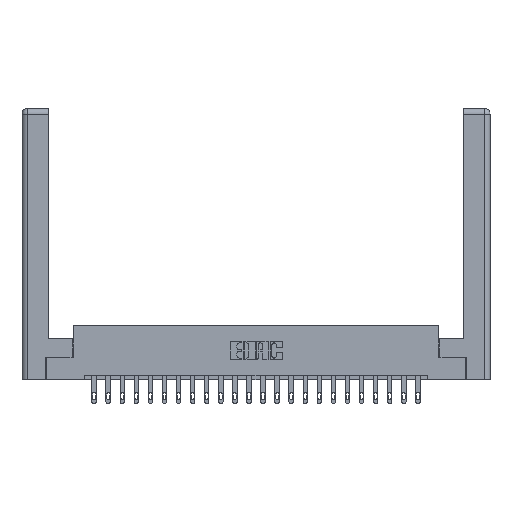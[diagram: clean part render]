
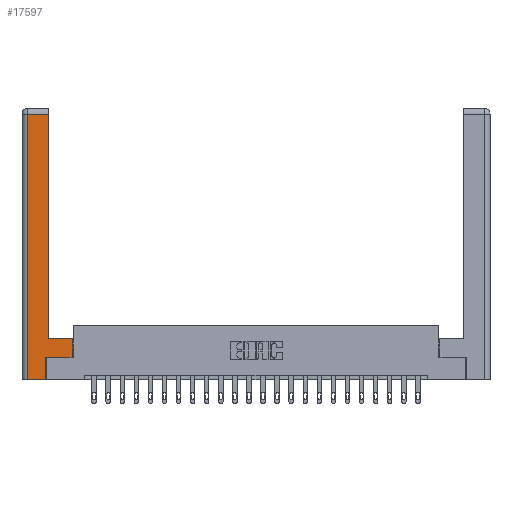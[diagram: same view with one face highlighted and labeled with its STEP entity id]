
A CAD part, top view. The second image highlights one B-rep face of the part: STEP entity #17597.
In plain terms, the highlighted planar face has unit normal (0, 0, 1).
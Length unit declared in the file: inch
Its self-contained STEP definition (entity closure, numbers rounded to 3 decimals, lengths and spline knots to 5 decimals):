
#208 = VECTOR ( 'NONE', #2813, 39.37008 ) ;
#710 = CARTESIAN_POINT ( 'NONE',  ( 0.565, 0.45, 0. ) ) ;
#1261 = VECTOR ( 'NONE', #11928, 39.37008 ) ;
#1658 = VERTEX_POINT ( 'NONE', #710 ) ;
#2043 = LINE ( 'NONE', #23170, #2915 ) ;
#2446 = DIRECTION ( 'NONE',  ( 0., 1., 0. ) ) ;
#2464 = VERTEX_POINT ( 'NONE', #9909 ) ;
#2813 = DIRECTION ( 'NONE',  ( 0., 1., 0. ) ) ;
#2915 = VECTOR ( 'NONE', #17894, 39.37008 ) ;
#3026 = EDGE_LOOP ( 'NONE', ( #8610, #19507, #13504, #21612, #8413, #15944, #18445, #5340 ) ) ;
#3492 = LINE ( 'NONE', #3715, #17320 ) ;
#3670 = VERTEX_POINT ( 'NONE', #4902 ) ;
#3715 = CARTESIAN_POINT ( 'NONE',  ( 0.265, 0., 0. ) ) ;
#3839 = EDGE_CURVE ( 'NONE', #1658, #21375, #17519, .T. ) ;
#3947 = CARTESIAN_POINT ( 'NONE',  ( 0.565, 0.45, 0. ) ) ;
#4124 = CARTESIAN_POINT ( 'NONE',  ( 0.295, 0.45, 0. ) ) ;
#4676 = LINE ( 'NONE', #12183, #22769 ) ;
#4801 = DIRECTION ( 'NONE',  ( -1., 0., 0. ) ) ;
#4902 = CARTESIAN_POINT ( 'NONE',  ( 0.295, 2.94, 0. ) ) ;
#5340 = ORIENTED_EDGE ( 'NONE', *, *, #3839, .T. ) ;
#5604 = CARTESIAN_POINT ( 'NONE',  ( 0.295, 0.45, 0. ) ) ;
#6064 = EDGE_CURVE ( 'NONE', #7318, #17657, #23118, .T. ) ;
#6409 = VERTEX_POINT ( 'NONE', #15928 ) ;
#6673 = DIRECTION ( 'NONE',  ( 1., 0., 0. ) ) ;
#6937 = VECTOR ( 'NONE', #2446, 39.37008 ) ;
#7318 = VERTEX_POINT ( 'NONE', #20897 ) ;
#7403 = FACE_OUTER_BOUND ( 'NONE', #3026, .T. ) ;
#8309 = CARTESIAN_POINT ( 'NONE',  ( 0.0615, 0., 0. ) ) ;
#8355 = EDGE_CURVE ( 'NONE', #2464, #1658, #20774, .T. ) ;
#8413 = ORIENTED_EDGE ( 'NONE', *, *, #6064, .T. ) ;
#8610 = ORIENTED_EDGE ( 'NONE', *, *, #10996, .T. ) ;
#9100 = EDGE_CURVE ( 'NONE', #6409, #7318, #3492, .T. ) ;
#9909 = CARTESIAN_POINT ( 'NONE',  ( 0.565, 0.245, 0. ) ) ;
#10368 = PLANE ( 'NONE',  #14100 ) ;
#10924 = LINE ( 'NONE', #8309, #1261 ) ;
#10996 = EDGE_CURVE ( 'NONE', #21375, #3670, #20335, .T. ) ;
#11390 = VECTOR ( 'NONE', #12776, 39.37008 ) ;
#11513 = CARTESIAN_POINT ( 'NONE',  ( 0., 0., 0. ) ) ;
#11928 = DIRECTION ( 'NONE',  ( 0., -1., 0. ) ) ;
#12183 = CARTESIAN_POINT ( 'NONE',  ( 0.0615, 2.94, 0. ) ) ;
#12776 = DIRECTION ( 'NONE',  ( 0., 1., 0. ) ) ;
#12834 = DIRECTION ( 'NONE',  ( 0., 0., -1. ) ) ;
#13333 = CARTESIAN_POINT ( 'NONE',  ( 0.295, 3., 0. ) ) ;
#13504 = ORIENTED_EDGE ( 'NONE', *, *, #20270, .T. ) ;
#13834 = CARTESIAN_POINT ( 'NONE',  ( 0.0615, 2.94, 0. ) ) ;
#14100 = AXIS2_PLACEMENT_3D ( 'NONE', #11513, #12834, #4801 ) ;
#15358 = CARTESIAN_POINT ( 'NONE',  ( 0.265, 0.245, 0. ) ) ;
#15503 = EDGE_CURVE ( 'NONE', #17657, #2464, #2043, .T. ) ;
#15928 = CARTESIAN_POINT ( 'NONE',  ( 0.0615, 0., 0. ) ) ;
#15944 = ORIENTED_EDGE ( 'NONE', *, *, #15503, .T. ) ;
#15970 = DIRECTION ( 'NONE',  ( -1., 0., 0. ) ) ;
#16846 = CARTESIAN_POINT ( 'NONE',  ( 0.265, 0.245, 0. ) ) ;
#17320 = VECTOR ( 'NONE', #6673, 39.37008 ) ;
#17519 = LINE ( 'NONE', #5604, #20934 ) ;
#17597 = ADVANCED_FACE ( 'NONE', ( #7403 ), #10368, .F. ) ;
#17657 = VERTEX_POINT ( 'NONE', #15358 ) ;
#17894 = DIRECTION ( 'NONE',  ( 1., 0., 0. ) ) ;
#18445 = ORIENTED_EDGE ( 'NONE', *, *, #8355, .T. ) ;
#19507 = ORIENTED_EDGE ( 'NONE', *, *, #20493, .T. ) ;
#20270 = EDGE_CURVE ( 'NONE', #20278, #6409, #10924, .T. ) ;
#20278 = VERTEX_POINT ( 'NONE', #13834 ) ;
#20335 = LINE ( 'NONE', #13333, #208 ) ;
#20493 = EDGE_CURVE ( 'NONE', #3670, #20278, #4676, .T. ) ;
#20774 = LINE ( 'NONE', #3947, #11390 ) ;
#20897 = CARTESIAN_POINT ( 'NONE',  ( 0.265, 0., 0. ) ) ;
#20934 = VECTOR ( 'NONE', #23373, 39.37008 ) ;
#21375 = VERTEX_POINT ( 'NONE', #4124 ) ;
#21612 = ORIENTED_EDGE ( 'NONE', *, *, #9100, .T. ) ;
#22769 = VECTOR ( 'NONE', #15970, 39.37008 ) ;
#23118 = LINE ( 'NONE', #16846, #6937 ) ;
#23170 = CARTESIAN_POINT ( 'NONE',  ( 0.565, 0.245, 0. ) ) ;
#23373 = DIRECTION ( 'NONE',  ( -1., 0., 0. ) ) ;
